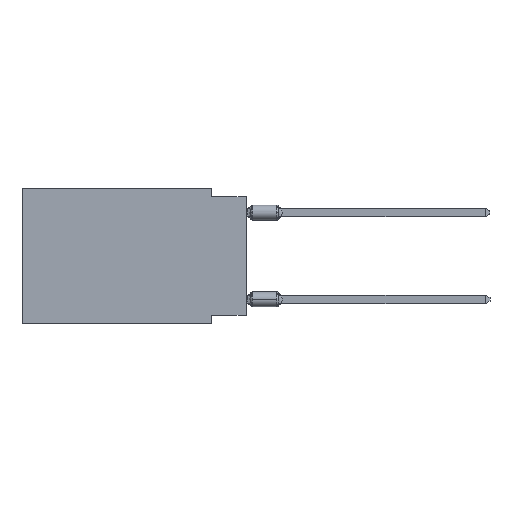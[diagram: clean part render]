
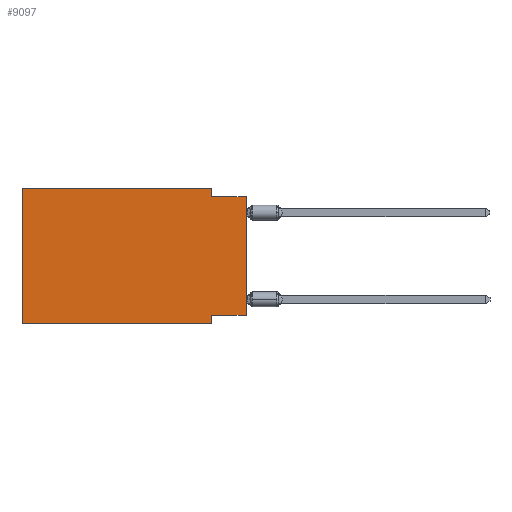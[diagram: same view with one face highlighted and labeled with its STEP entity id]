
A CAD part, left-side view. The second image highlights one B-rep face of the part: STEP entity #9097.
In plain terms, the highlighted planar face has unit normal (-1, 0, 0).
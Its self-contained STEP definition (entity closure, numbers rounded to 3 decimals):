
#521 = LINE ( 'NONE', #2044, #1675 ) ;
#649 = VERTEX_POINT ( 'NONE', #8896 ) ;
#886 = VERTEX_POINT ( 'NONE', #17792 ) ;
#1160 = DIRECTION ( 'NONE',  ( 1., 0., 0. ) ) ;
#1281 = CARTESIAN_POINT ( 'NONE',  ( 0., 0., 0. ) ) ;
#1616 = LINE ( 'NONE', #7339, #10761 ) ;
#1675 = VECTOR ( 'NONE', #6278, 1000. ) ;
#2044 = CARTESIAN_POINT ( 'NONE',  ( 0., 16.383, 0. ) ) ;
#2194 = ORIENTED_EDGE ( 'NONE', *, *, #5328, .F. ) ;
#2752 = ORIENTED_EDGE ( 'NONE', *, *, #9811, .F. ) ;
#3298 = LINE ( 'NONE', #13337, #16215 ) ;
#3513 = LINE ( 'NONE', #6141, #12605 ) ;
#4181 = DIRECTION ( 'NONE',  ( 0., 0., -1. ) ) ;
#4238 = VECTOR ( 'NONE', #8724, 1000. ) ;
#4388 = VECTOR ( 'NONE', #13474, 1000. ) ;
#5328 = EDGE_CURVE ( 'NONE', #16340, #649, #3298, .T. ) ;
#5403 = FACE_OUTER_BOUND ( 'NONE', #11595, .T. ) ;
#5420 = VERTEX_POINT ( 'NONE', #9558 ) ;
#6113 = LINE ( 'NONE', #13531, #17369 ) ;
#6141 = CARTESIAN_POINT ( 'NONE',  ( 0., 0., -9.271 ) ) ;
#6278 = DIRECTION ( 'NONE',  ( 0., 0., 1. ) ) ;
#7123 = EDGE_CURVE ( 'NONE', #5420, #18040, #12933, .T. ) ;
#7124 = ORIENTED_EDGE ( 'NONE', *, *, #7123, .T. ) ;
#7339 = CARTESIAN_POINT ( 'NONE',  ( 0., 2.54, -9.906 ) ) ;
#7451 = VERTEX_POINT ( 'NONE', #8305 ) ;
#7693 = DIRECTION ( 'NONE',  ( 0., 0., -1. ) ) ;
#7773 = ORIENTED_EDGE ( 'NONE', *, *, #11655, .F. ) ;
#8305 = CARTESIAN_POINT ( 'NONE',  ( 0., 2.54, -9.271 ) ) ;
#8325 = ORIENTED_EDGE ( 'NONE', *, *, #18083, .F. ) ;
#8361 = EDGE_CURVE ( 'NONE', #886, #11356, #15865, .T. ) ;
#8724 = DIRECTION ( 'NONE',  ( 0., -1., 0. ) ) ;
#8896 = CARTESIAN_POINT ( 'NONE',  ( 0., 2.54, -0.635 ) ) ;
#9046 = CARTESIAN_POINT ( 'NONE',  ( 0., 0., -0.635 ) ) ;
#9097 = ADVANCED_FACE ( 'NONE', ( #5403 ), #10835, .F. ) ;
#9305 = EDGE_CURVE ( 'NONE', #7451, #11356, #1616, .T. ) ;
#9558 = CARTESIAN_POINT ( 'NONE',  ( 0., 0., -9.271 ) ) ;
#9811 = EDGE_CURVE ( 'NONE', #649, #18040, #6113, .T. ) ;
#9938 = CARTESIAN_POINT ( 'NONE',  ( 0., 16.383, 0. ) ) ;
#10449 = AXIS2_PLACEMENT_3D ( 'NONE', #15235, #1160, #13937 ) ;
#10598 = DIRECTION ( 'NONE',  ( 0., -1., 0. ) ) ;
#10602 = EDGE_CURVE ( 'NONE', #5420, #7451, #3513, .T. ) ;
#10761 = VECTOR ( 'NONE', #4181, 1000. ) ;
#10835 = PLANE ( 'NONE',  #10449 ) ;
#11356 = VERTEX_POINT ( 'NONE', #12488 ) ;
#11595 = EDGE_LOOP ( 'NONE', ( #7124, #2752, #2194, #8325, #7773, #17238, #12018, #11964 ) ) ;
#11655 = EDGE_CURVE ( 'NONE', #886, #12708, #521, .T. ) ;
#11801 = CARTESIAN_POINT ( 'NONE',  ( 0., 2.54, 0. ) ) ;
#11964 = ORIENTED_EDGE ( 'NONE', *, *, #10602, .F. ) ;
#12018 = ORIENTED_EDGE ( 'NONE', *, *, #9305, .F. ) ;
#12154 = CARTESIAN_POINT ( 'NONE',  ( 0., 16.383, 0. ) ) ;
#12245 = LINE ( 'NONE', #12154, #4388 ) ;
#12488 = CARTESIAN_POINT ( 'NONE',  ( 0., 2.54, -9.906 ) ) ;
#12605 = VECTOR ( 'NONE', #16077, 1000. ) ;
#12708 = VERTEX_POINT ( 'NONE', #9938 ) ;
#12790 = CARTESIAN_POINT ( 'NONE',  ( 0., 16.383, -9.906 ) ) ;
#12933 = LINE ( 'NONE', #1281, #16769 ) ;
#13122 = DIRECTION ( 'NONE',  ( 0., 0., 1. ) ) ;
#13337 = CARTESIAN_POINT ( 'NONE',  ( 0., 2.54, 0. ) ) ;
#13474 = DIRECTION ( 'NONE',  ( 0., -1., 0. ) ) ;
#13531 = CARTESIAN_POINT ( 'NONE',  ( 0., 0., -0.635 ) ) ;
#13937 = DIRECTION ( 'NONE',  ( 0., 0., -1. ) ) ;
#15235 = CARTESIAN_POINT ( 'NONE',  ( 0., 16.383, 0. ) ) ;
#15865 = LINE ( 'NONE', #12790, #4238 ) ;
#16077 = DIRECTION ( 'NONE',  ( 0., 1., 0. ) ) ;
#16215 = VECTOR ( 'NONE', #7693, 1000. ) ;
#16340 = VERTEX_POINT ( 'NONE', #11801 ) ;
#16769 = VECTOR ( 'NONE', #13122, 1000. ) ;
#17238 = ORIENTED_EDGE ( 'NONE', *, *, #8361, .T. ) ;
#17369 = VECTOR ( 'NONE', #10598, 1000. ) ;
#17792 = CARTESIAN_POINT ( 'NONE',  ( 0., 16.383, -9.906 ) ) ;
#18040 = VERTEX_POINT ( 'NONE', #9046 ) ;
#18083 = EDGE_CURVE ( 'NONE', #12708, #16340, #12245, .T. ) ;
